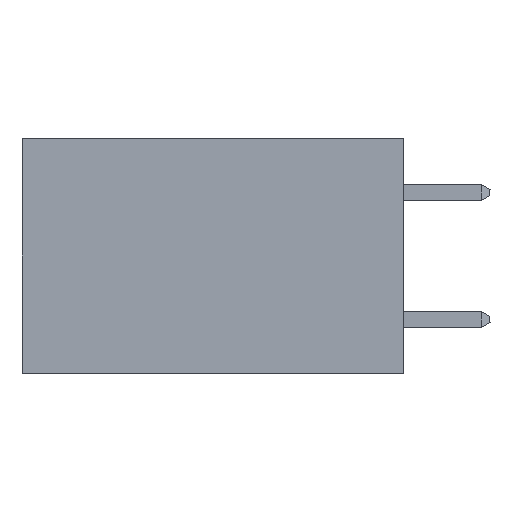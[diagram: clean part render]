
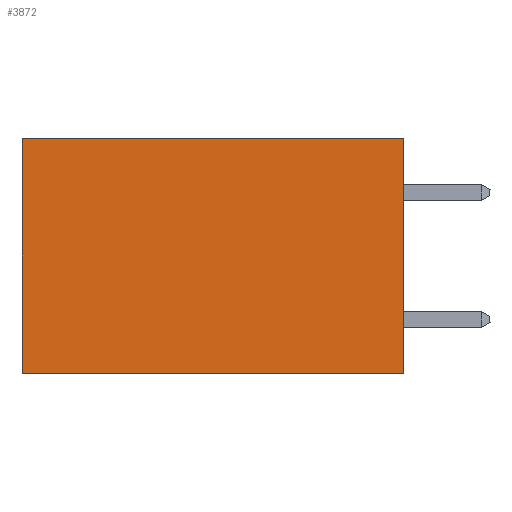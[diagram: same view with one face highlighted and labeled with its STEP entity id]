
A CAD part, left-side view. The second image highlights one B-rep face of the part: STEP entity #3872.
In plain terms, the highlighted planar face has unit normal (-1, 0, 0).
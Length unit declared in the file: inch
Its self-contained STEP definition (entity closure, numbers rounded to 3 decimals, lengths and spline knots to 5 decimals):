
#1061 = ORIENTED_EDGE ( 'NONE', *, *, #6639, .T. ) ;
#1458 = FACE_OUTER_BOUND ( 'NONE', #8902, .T. ) ;
#1466 = EDGE_CURVE ( 'NONE', #8720, #8692, #9009, .T. ) ;
#1524 = DIRECTION ( 'NONE',  ( 0., 0., -1. ) ) ;
#1552 = DIRECTION ( 'NONE',  ( 1., 0., 0. ) ) ;
#1644 = VECTOR ( 'NONE', #2144, 39.37008 ) ;
#1986 = ORIENTED_EDGE ( 'NONE', *, *, #4249, .F. ) ;
#2000 = VECTOR ( 'NONE', #7168, 39.37008 ) ;
#2038 = ORIENTED_EDGE ( 'NONE', *, *, #1466, .F. ) ;
#2144 = DIRECTION ( 'NONE',  ( 0., 1., 0. ) ) ;
#2318 = CARTESIAN_POINT ( 'NONE',  ( 0.2875, 0., -0.37 ) ) ;
#2747 = CARTESIAN_POINT ( 'NONE',  ( 0.2875, 0.6, 0. ) ) ;
#3631 = LINE ( 'NONE', #6016, #1644 ) ;
#3718 = CARTESIAN_POINT ( 'NONE',  ( 0.2875, 0.6, -0.37 ) ) ;
#3872 = ADVANCED_FACE ( 'NONE', ( #1458 ), #4185, .F. ) ;
#3894 = CARTESIAN_POINT ( 'NONE',  ( 0.2875, 0., 0. ) ) ;
#4185 = PLANE ( 'NONE',  #8157 ) ;
#4249 = EDGE_CURVE ( 'NONE', #7383, #8720, #8240, .T. ) ;
#5085 = DIRECTION ( 'NONE',  ( 0., 1., 0. ) ) ;
#5254 = VECTOR ( 'NONE', #5085, 39.37008 ) ;
#5987 = VECTOR ( 'NONE', #6415, 39.37008 ) ;
#6016 = CARTESIAN_POINT ( 'NONE',  ( 0.2875, 0., 0. ) ) ;
#6168 = EDGE_CURVE ( 'NONE', #7383, #6943, #3631, .T. ) ;
#6319 = ORIENTED_EDGE ( 'NONE', *, *, #6168, .T. ) ;
#6415 = DIRECTION ( 'NONE',  ( 0., 0., -1. ) ) ;
#6545 = CARTESIAN_POINT ( 'NONE',  ( 0.2875, 0.6, 0. ) ) ;
#6615 = CARTESIAN_POINT ( 'NONE',  ( 0.2875, 0., -0.37 ) ) ;
#6639 = EDGE_CURVE ( 'NONE', #6943, #8692, #8099, .T. ) ;
#6943 = VERTEX_POINT ( 'NONE', #6545 ) ;
#7168 = DIRECTION ( 'NONE',  ( 0., 0., -1. ) ) ;
#7178 = CARTESIAN_POINT ( 'NONE',  ( 0.2875, 0., 0. ) ) ;
#7203 = CARTESIAN_POINT ( 'NONE',  ( 0.2875, 0., 0. ) ) ;
#7383 = VERTEX_POINT ( 'NONE', #7178 ) ;
#8099 = LINE ( 'NONE', #2747, #5987 ) ;
#8157 = AXIS2_PLACEMENT_3D ( 'NONE', #3894, #1552, #1524 ) ;
#8240 = LINE ( 'NONE', #7203, #2000 ) ;
#8692 = VERTEX_POINT ( 'NONE', #3718 ) ;
#8720 = VERTEX_POINT ( 'NONE', #6615 ) ;
#8902 = EDGE_LOOP ( 'NONE', ( #1061, #2038, #1986, #6319 ) ) ;
#9009 = LINE ( 'NONE', #2318, #5254 ) ;
